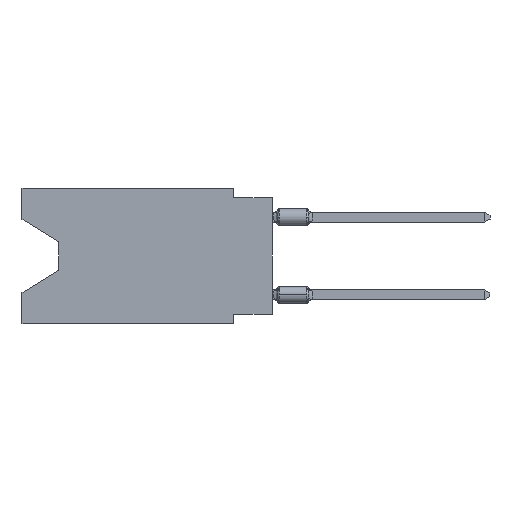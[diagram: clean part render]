
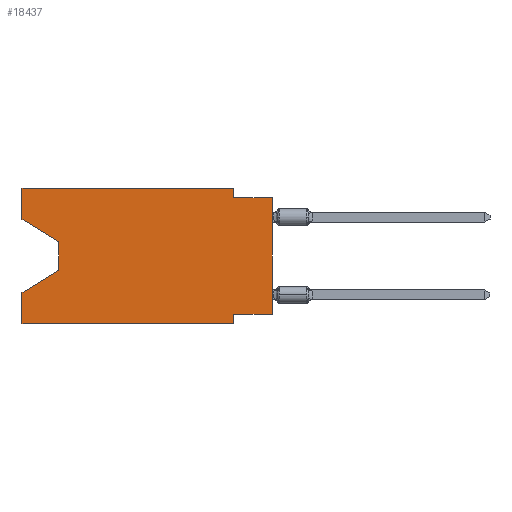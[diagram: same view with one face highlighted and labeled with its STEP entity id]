
A CAD part, left-side view. The second image highlights one B-rep face of the part: STEP entity #18437.
In plain terms, the highlighted planar face has unit normal (-1, 0, 0).
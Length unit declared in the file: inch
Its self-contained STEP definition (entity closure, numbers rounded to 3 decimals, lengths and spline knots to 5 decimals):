
#125 = DIRECTION ( 'NONE',  ( 0., 0.855, -0.519 ) ) ;
#346 = LINE ( 'NONE', #17034, #11819 ) ;
#656 = EDGE_CURVE ( 'NONE', #10077, #2256, #10281, .T. ) ;
#927 = DIRECTION ( 'NONE',  ( 0., 0., 1. ) ) ;
#1002 = VECTOR ( 'NONE', #11833, 39.37008 ) ;
#1285 = VECTOR ( 'NONE', #4968, 39.37008 ) ;
#1455 = CARTESIAN_POINT ( 'NONE',  ( 0., 0.645, 0. ) ) ;
#1827 = LINE ( 'NONE', #18790, #1285 ) ;
#2212 = EDGE_CURVE ( 'NONE', #2256, #19009, #8122, .T. ) ;
#2256 = VERTEX_POINT ( 'NONE', #17501 ) ;
#2666 = PLANE ( 'NONE',  #11516 ) ;
#2685 = EDGE_CURVE ( 'NONE', #6164, #13049, #1827, .T. ) ;
#2735 = VECTOR ( 'NONE', #13074, 39.37008 ) ;
#2993 = VECTOR ( 'NONE', #3435, 39.37008 ) ;
#3152 = CARTESIAN_POINT ( 'NONE',  ( 0., 0., -0.025 ) ) ;
#3158 = LINE ( 'NONE', #3250, #4621 ) ;
#3250 = CARTESIAN_POINT ( 'NONE',  ( 0., 0.55, -0.212 ) ) ;
#3266 = VERTEX_POINT ( 'NONE', #6481 ) ;
#3435 = DIRECTION ( 'NONE',  ( 0., 0., -1. ) ) ;
#3590 = LINE ( 'NONE', #18947, #18212 ) ;
#3699 = ORIENTED_EDGE ( 'NONE', *, *, #13114, .T. ) ;
#4046 = LINE ( 'NONE', #7096, #9413 ) ;
#4621 = VECTOR ( 'NONE', #125, 39.37008 ) ;
#4968 = DIRECTION ( 'NONE',  ( 0., 1., 0. ) ) ;
#4969 = LINE ( 'NONE', #8595, #5231 ) ;
#5167 = ORIENTED_EDGE ( 'NONE', *, *, #17368, .F. ) ;
#5231 = VECTOR ( 'NONE', #16282, 39.37008 ) ;
#5575 = LINE ( 'NONE', #13277, #1002 ) ;
#6164 = VERTEX_POINT ( 'NONE', #13978 ) ;
#6307 = DIRECTION ( 'NONE',  ( 0., 0., -1. ) ) ;
#6475 = LINE ( 'NONE', #15792, #2993 ) ;
#6481 = CARTESIAN_POINT ( 'NONE',  ( 0., 0.645, -0.26975 ) ) ;
#7096 = CARTESIAN_POINT ( 'NONE',  ( 0., 0.645, 0. ) ) ;
#7181 = VERTEX_POINT ( 'NONE', #14990 ) ;
#7442 = CARTESIAN_POINT ( 'NONE',  ( 0., 0.645, -0.08025 ) ) ;
#8122 = LINE ( 'NONE', #9936, #19675 ) ;
#8475 = CARTESIAN_POINT ( 'NONE',  ( 0., 0.1, 0. ) ) ;
#8595 = CARTESIAN_POINT ( 'NONE',  ( 0., 0., 0. ) ) ;
#8635 = VECTOR ( 'NONE', #10392, 39.37008 ) ;
#8843 = DIRECTION ( 'NONE',  ( 1., 0., 0. ) ) ;
#8867 = VERTEX_POINT ( 'NONE', #3152 ) ;
#8900 = EDGE_CURVE ( 'NONE', #6164, #8867, #4969, .T. ) ;
#8978 = LINE ( 'NONE', #10488, #8635 ) ;
#9383 = ORIENTED_EDGE ( 'NONE', *, *, #13476, .F. ) ;
#9398 = EDGE_CURVE ( 'NONE', #12676, #7181, #6475, .T. ) ;
#9413 = VECTOR ( 'NONE', #927, 39.37008 ) ;
#9868 = DIRECTION ( 'NONE',  ( 0., -1., 0. ) ) ;
#9936 = CARTESIAN_POINT ( 'NONE',  ( 0., 0.645, 0. ) ) ;
#9978 = ORIENTED_EDGE ( 'NONE', *, *, #9398, .T. ) ;
#10073 = DIRECTION ( 'NONE',  ( 0., 0., 1. ) ) ;
#10077 = VERTEX_POINT ( 'NONE', #7442 ) ;
#10230 = CARTESIAN_POINT ( 'NONE',  ( 0., 0.55, -0.138 ) ) ;
#10281 = LINE ( 'NONE', #19041, #18045 ) ;
#10303 = EDGE_CURVE ( 'NONE', #10077, #12676, #19409, .T. ) ;
#10323 = ORIENTED_EDGE ( 'NONE', *, *, #8900, .T. ) ;
#10392 = DIRECTION ( 'NONE',  ( 0., -1., 0. ) ) ;
#10488 = CARTESIAN_POINT ( 'NONE',  ( 0., 0., -0.025 ) ) ;
#11476 = CARTESIAN_POINT ( 'NONE',  ( 0., 0.645, -0.35 ) ) ;
#11516 = AXIS2_PLACEMENT_3D ( 'NONE', #1455, #8843, #15018 ) ;
#11819 = VECTOR ( 'NONE', #6307, 39.37008 ) ;
#11833 = DIRECTION ( 'NONE',  ( 0., 0., -1. ) ) ;
#11973 = FACE_OUTER_BOUND ( 'NONE', #17863, .T. ) ;
#12176 = CARTESIAN_POINT ( 'NONE',  ( 0., 0.1, -0.025 ) ) ;
#12676 = VERTEX_POINT ( 'NONE', #10230 ) ;
#12790 = ORIENTED_EDGE ( 'NONE', *, *, #13479, .F. ) ;
#13049 = VERTEX_POINT ( 'NONE', #19173 ) ;
#13074 = DIRECTION ( 'NONE',  ( 0., -0.855, -0.519 ) ) ;
#13114 = EDGE_CURVE ( 'NONE', #16944, #13184, #3590, .T. ) ;
#13184 = VERTEX_POINT ( 'NONE', #14832 ) ;
#13277 = CARTESIAN_POINT ( 'NONE',  ( 0., 0.1, -0.35 ) ) ;
#13473 = CARTESIAN_POINT ( 'NONE',  ( 0., 0.645, -0.08025 ) ) ;
#13476 = EDGE_CURVE ( 'NONE', #16944, #3266, #4046, .T. ) ;
#13479 = EDGE_CURVE ( 'NONE', #13049, #13184, #5575, .T. ) ;
#13978 = CARTESIAN_POINT ( 'NONE',  ( 0., 0., -0.325 ) ) ;
#14805 = ORIENTED_EDGE ( 'NONE', *, *, #2685, .F. ) ;
#14832 = CARTESIAN_POINT ( 'NONE',  ( 0., 0.1, -0.35 ) ) ;
#14990 = CARTESIAN_POINT ( 'NONE',  ( 0., 0.55, -0.212 ) ) ;
#15018 = DIRECTION ( 'NONE',  ( 0., 0., -1. ) ) ;
#15025 = ORIENTED_EDGE ( 'NONE', *, *, #2212, .F. ) ;
#15719 = EDGE_CURVE ( 'NONE', #7181, #3266, #3158, .T. ) ;
#15792 = CARTESIAN_POINT ( 'NONE',  ( 0., 0.55, -0.138 ) ) ;
#16108 = ORIENTED_EDGE ( 'NONE', *, *, #10303, .T. ) ;
#16282 = DIRECTION ( 'NONE',  ( 0., 0., 1. ) ) ;
#16944 = VERTEX_POINT ( 'NONE', #11476 ) ;
#17034 = CARTESIAN_POINT ( 'NONE',  ( 0., 0.1, 0. ) ) ;
#17368 = EDGE_CURVE ( 'NONE', #19009, #19731, #346, .T. ) ;
#17501 = CARTESIAN_POINT ( 'NONE',  ( 0., 0.645, 0. ) ) ;
#17701 = DIRECTION ( 'NONE',  ( 0., -1., 0. ) ) ;
#17798 = ORIENTED_EDGE ( 'NONE', *, *, #656, .F. ) ;
#17840 = ORIENTED_EDGE ( 'NONE', *, *, #19182, .F. ) ;
#17863 = EDGE_LOOP ( 'NONE', ( #16108, #9978, #18030, #9383, #3699, #12790, #14805, #10323, #17840, #5167, #15025, #17798 ) ) ;
#18030 = ORIENTED_EDGE ( 'NONE', *, *, #15719, .T. ) ;
#18045 = VECTOR ( 'NONE', #10073, 39.37008 ) ;
#18212 = VECTOR ( 'NONE', #9868, 39.37008 ) ;
#18437 = ADVANCED_FACE ( 'NONE', ( #11973 ), #2666, .F. ) ;
#18790 = CARTESIAN_POINT ( 'NONE',  ( 0., 0., -0.325 ) ) ;
#18947 = CARTESIAN_POINT ( 'NONE',  ( 0., 0.645, -0.35 ) ) ;
#19009 = VERTEX_POINT ( 'NONE', #8475 ) ;
#19041 = CARTESIAN_POINT ( 'NONE',  ( 0., 0.645, 0. ) ) ;
#19173 = CARTESIAN_POINT ( 'NONE',  ( 0., 0.1, -0.325 ) ) ;
#19182 = EDGE_CURVE ( 'NONE', #19731, #8867, #8978, .T. ) ;
#19409 = LINE ( 'NONE', #13473, #2735 ) ;
#19675 = VECTOR ( 'NONE', #17701, 39.37008 ) ;
#19731 = VERTEX_POINT ( 'NONE', #12176 ) ;
